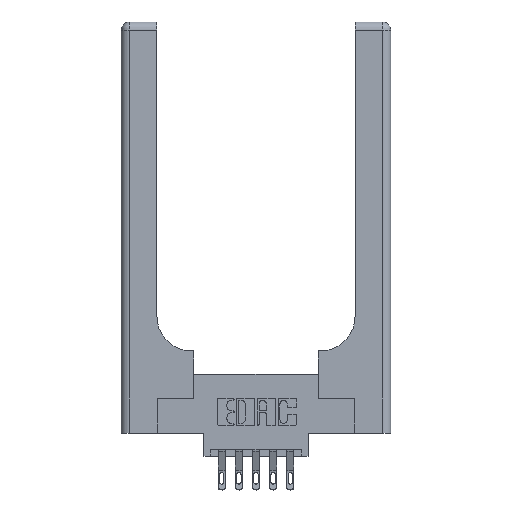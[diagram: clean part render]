
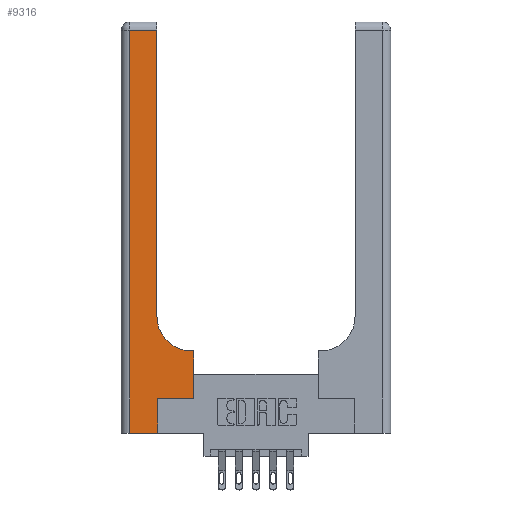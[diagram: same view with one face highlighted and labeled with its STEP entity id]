
A CAD part, top view. The second image highlights one B-rep face of the part: STEP entity #9316.
In plain terms, the highlighted planar face has unit normal (0, 0, 1).
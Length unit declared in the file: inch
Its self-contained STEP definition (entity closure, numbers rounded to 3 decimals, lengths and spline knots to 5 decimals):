
#167 = VERTEX_POINT ( 'NONE', #4563 ) ;
#323 = EDGE_CURVE ( 'NONE', #3433, #5464, #5921, .T. ) ;
#643 = ORIENTED_EDGE ( 'NONE', *, *, #5750, .T. ) ;
#993 = LINE ( 'NONE', #2017, #3106 ) ;
#1032 = CARTESIAN_POINT ( 'NONE',  ( 0., 2.94, 0.37 ) ) ;
#1256 = DIRECTION ( 'NONE',  ( 0., 1., 0. ) ) ;
#1397 = CARTESIAN_POINT ( 'NONE',  ( 0., 0., 0.37 ) ) ;
#1846 = AXIS2_PLACEMENT_3D ( 'NONE', #10716, #11655, #9617 ) ;
#2014 = ORIENTED_EDGE ( 'NONE', *, *, #12668, .T. ) ;
#2017 = CARTESIAN_POINT ( 'NONE',  ( 0.265, 0., 0.37 ) ) ;
#2344 = CARTESIAN_POINT ( 'NONE',  ( 0.528, 0.25, 0.37 ) ) ;
#2393 = CARTESIAN_POINT ( 'NONE',  ( 0.26, 0.85, 0.37 ) ) ;
#2471 = VERTEX_POINT ( 'NONE', #9670 ) ;
#2519 = VERTEX_POINT ( 'NONE', #8595 ) ;
#2969 = FACE_OUTER_BOUND ( 'NONE', #3554, .T. ) ;
#3106 = VECTOR ( 'NONE', #5424, 39.37008 ) ;
#3239 = ORIENTED_EDGE ( 'NONE', *, *, #13662, .T. ) ;
#3306 = VECTOR ( 'NONE', #1256, 39.37008 ) ;
#3320 = EDGE_CURVE ( 'NONE', #2519, #10073, #5226, .T. ) ;
#3433 = VERTEX_POINT ( 'NONE', #2393 ) ;
#3554 = EDGE_LOOP ( 'NONE', ( #11890, #8888, #4385, #13176, #3239, #643, #4139, #2014, #13014 ) ) ;
#3565 = CARTESIAN_POINT ( 'NONE',  ( 0.26, 3., 0.37 ) ) ;
#3629 = VECTOR ( 'NONE', #10874, 39.37008 ) ;
#4048 = CARTESIAN_POINT ( 'NONE',  ( 0.51, 0.85, 0.37 ) ) ;
#4139 = ORIENTED_EDGE ( 'NONE', *, *, #11476, .T. ) ;
#4223 = EDGE_CURVE ( 'NONE', #10073, #14214, #12336, .T. ) ;
#4385 = ORIENTED_EDGE ( 'NONE', *, *, #3320, .T. ) ;
#4544 = CARTESIAN_POINT ( 'NONE',  ( 0.06, 0., 0.37 ) ) ;
#4563 = CARTESIAN_POINT ( 'NONE',  ( 0.51, 0.6, 0.37 ) ) ;
#5118 = VECTOR ( 'NONE', #11039, 39.37008 ) ;
#5226 = LINE ( 'NONE', #8553, #3629 ) ;
#5424 = DIRECTION ( 'NONE',  ( 0., 1., 0. ) ) ;
#5464 = VERTEX_POINT ( 'NONE', #11771 ) ;
#5508 = VERTEX_POINT ( 'NONE', #7290 ) ;
#5542 = LINE ( 'NONE', #11984, #11166 ) ;
#5750 = EDGE_CURVE ( 'NONE', #5508, #2471, #9142, .T. ) ;
#5921 = LINE ( 'NONE', #3565, #8674 ) ;
#6180 = CARTESIAN_POINT ( 'NONE',  ( 0.265, 0., 0.37 ) ) ;
#6235 = VECTOR ( 'NONE', #8928, 39.37008 ) ;
#6399 = LINE ( 'NONE', #1032, #5118 ) ;
#6664 = VERTEX_POINT ( 'NONE', #11443 ) ;
#7290 = CARTESIAN_POINT ( 'NONE',  ( 0.265, 0.25, 0.37 ) ) ;
#8452 = DIRECTION ( 'NONE',  ( 1., 0., 0. ) ) ;
#8553 = CARTESIAN_POINT ( 'NONE',  ( 0.06, 3., 0.37 ) ) ;
#8595 = CARTESIAN_POINT ( 'NONE',  ( 0.06, 2.94, 0.37 ) ) ;
#8633 = EDGE_CURVE ( 'NONE', #167, #3433, #12005, .T. ) ;
#8674 = VECTOR ( 'NONE', #10287, 39.37008 ) ;
#8888 = ORIENTED_EDGE ( 'NONE', *, *, #10347, .T. ) ;
#8928 = DIRECTION ( 'NONE',  ( 1., 0., 0. ) ) ;
#9142 = LINE ( 'NONE', #9203, #10596 ) ;
#9203 = CARTESIAN_POINT ( 'NONE',  ( 0.265, 0.25, 0.37 ) ) ;
#9316 = ADVANCED_FACE ( 'NONE', ( #2969 ), #10498, .F. ) ;
#9617 = DIRECTION ( 'NONE',  ( -1., 0., 0. ) ) ;
#9670 = CARTESIAN_POINT ( 'NONE',  ( 0.528, 0.25, 0.37 ) ) ;
#10073 = VERTEX_POINT ( 'NONE', #4544 ) ;
#10287 = DIRECTION ( 'NONE',  ( 0., 1., 0. ) ) ;
#10347 = EDGE_CURVE ( 'NONE', #5464, #2519, #6399, .T. ) ;
#10387 = AXIS2_PLACEMENT_3D ( 'NONE', #4048, #10479, #8452 ) ;
#10479 = DIRECTION ( 'NONE',  ( 0., 0., -1. ) ) ;
#10498 = PLANE ( 'NONE',  #1846 ) ;
#10596 = VECTOR ( 'NONE', #13565, 39.37008 ) ;
#10716 = CARTESIAN_POINT ( 'NONE',  ( 0., 3., 0.37 ) ) ;
#10874 = DIRECTION ( 'NONE',  ( 0., -1., 0. ) ) ;
#11039 = DIRECTION ( 'NONE',  ( -1., 0., 0. ) ) ;
#11166 = VECTOR ( 'NONE', #12933, 39.37008 ) ;
#11261 = LINE ( 'NONE', #2344, #3306 ) ;
#11443 = CARTESIAN_POINT ( 'NONE',  ( 0.528, 0.6, 0.37 ) ) ;
#11476 = EDGE_CURVE ( 'NONE', #2471, #6664, #11261, .T. ) ;
#11655 = DIRECTION ( 'NONE',  ( 0., 0., -1. ) ) ;
#11771 = CARTESIAN_POINT ( 'NONE',  ( 0.26, 2.94, 0.37 ) ) ;
#11890 = ORIENTED_EDGE ( 'NONE', *, *, #323, .T. ) ;
#11984 = CARTESIAN_POINT ( 'NONE',  ( 0.26, 0.6, 0.37 ) ) ;
#12005 = CIRCLE ( 'NONE', #10387, 0.25 ) ;
#12336 = LINE ( 'NONE', #1397, #6235 ) ;
#12668 = EDGE_CURVE ( 'NONE', #6664, #167, #5542, .T. ) ;
#12933 = DIRECTION ( 'NONE',  ( -1., 0., 0. ) ) ;
#13014 = ORIENTED_EDGE ( 'NONE', *, *, #8633, .T. ) ;
#13176 = ORIENTED_EDGE ( 'NONE', *, *, #4223, .T. ) ;
#13565 = DIRECTION ( 'NONE',  ( 1., 0., 0. ) ) ;
#13662 = EDGE_CURVE ( 'NONE', #14214, #5508, #993, .T. ) ;
#14214 = VERTEX_POINT ( 'NONE', #6180 ) ;
